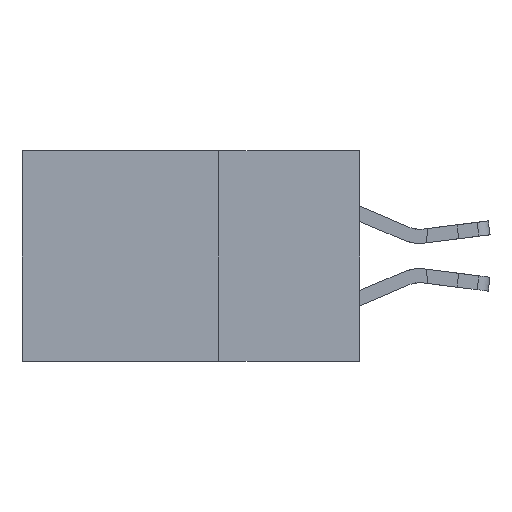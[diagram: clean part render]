
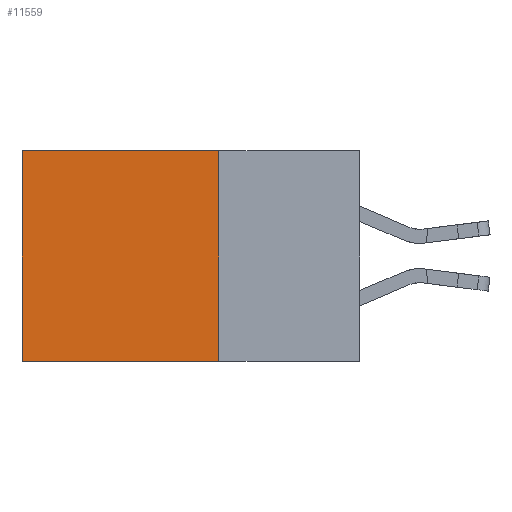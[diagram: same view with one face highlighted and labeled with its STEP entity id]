
A CAD part, left-side view. The second image highlights one B-rep face of the part: STEP entity #11559.
In plain terms, the highlighted planar face has unit normal (-1, 0, 0).
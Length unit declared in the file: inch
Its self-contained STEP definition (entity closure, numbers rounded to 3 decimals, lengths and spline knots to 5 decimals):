
#140 = EDGE_LOOP ( 'NONE', ( #3931, #13131, #12339, #5753 ) ) ;
#1578 = VECTOR ( 'NONE', #5965, 39.37008 ) ;
#1666 = CARTESIAN_POINT ( 'NONE',  ( 0.2875, 0.6, -0.375 ) ) ;
#1888 = LINE ( 'NONE', #8616, #3227 ) ;
#2150 = EDGE_CURVE ( 'NONE', #5075, #6208, #1888, .T. ) ;
#2804 = VECTOR ( 'NONE', #7892, 39.37008 ) ;
#3227 = VECTOR ( 'NONE', #11875, 39.37008 ) ;
#3515 = CARTESIAN_POINT ( 'NONE',  ( 0.2875, 0.25, -0.375 ) ) ;
#3803 = EDGE_CURVE ( 'NONE', #5177, #6208, #11381, .T. ) ;
#3931 = ORIENTED_EDGE ( 'NONE', *, *, #3803, .T. ) ;
#4137 = LINE ( 'NONE', #11536, #4879 ) ;
#4879 = VECTOR ( 'NONE', #5123, 39.37008 ) ;
#5075 = VERTEX_POINT ( 'NONE', #3515 ) ;
#5123 = DIRECTION ( 'NONE',  ( 0., 1., 0. ) ) ;
#5177 = VERTEX_POINT ( 'NONE', #13651 ) ;
#5753 = ORIENTED_EDGE ( 'NONE', *, *, #7704, .T. ) ;
#5810 = CARTESIAN_POINT ( 'NONE',  ( 0.2875, 0.25, -0.375 ) ) ;
#5965 = DIRECTION ( 'NONE',  ( 0., 0., -1. ) ) ;
#6208 = VERTEX_POINT ( 'NONE', #7348 ) ;
#6747 = LINE ( 'NONE', #5810, #2804 ) ;
#6864 = PLANE ( 'NONE',  #8631 ) ;
#7348 = CARTESIAN_POINT ( 'NONE',  ( 0.2875, 0.6, -0.375 ) ) ;
#7704 = EDGE_CURVE ( 'NONE', #9896, #5177, #4137, .T. ) ;
#7892 = DIRECTION ( 'NONE',  ( 0., 0., -1. ) ) ;
#7935 = DIRECTION ( 'NONE',  ( 1., 0., 0. ) ) ;
#8616 = CARTESIAN_POINT ( 'NONE',  ( 0.2875, 0.25, -0.375 ) ) ;
#8631 = AXIS2_PLACEMENT_3D ( 'NONE', #9068, #7935, #13251 ) ;
#9068 = CARTESIAN_POINT ( 'NONE',  ( 0.2875, 0.25, -0.375 ) ) ;
#9227 = CARTESIAN_POINT ( 'NONE',  ( 0.2875, 0.25, 0. ) ) ;
#9896 = VERTEX_POINT ( 'NONE', #9227 ) ;
#11381 = LINE ( 'NONE', #1666, #1578 ) ;
#11536 = CARTESIAN_POINT ( 'NONE',  ( 0.2875, 0.25, 0. ) ) ;
#11559 = ADVANCED_FACE ( 'NONE', ( #12110 ), #6864, .F. ) ;
#11875 = DIRECTION ( 'NONE',  ( 0., 1., 0. ) ) ;
#12110 = FACE_OUTER_BOUND ( 'NONE', #140, .T. ) ;
#12339 = ORIENTED_EDGE ( 'NONE', *, *, #13713, .F. ) ;
#13131 = ORIENTED_EDGE ( 'NONE', *, *, #2150, .F. ) ;
#13251 = DIRECTION ( 'NONE',  ( 0., 0., -1. ) ) ;
#13651 = CARTESIAN_POINT ( 'NONE',  ( 0.2875, 0.6, 0. ) ) ;
#13713 = EDGE_CURVE ( 'NONE', #9896, #5075, #6747, .T. ) ;
